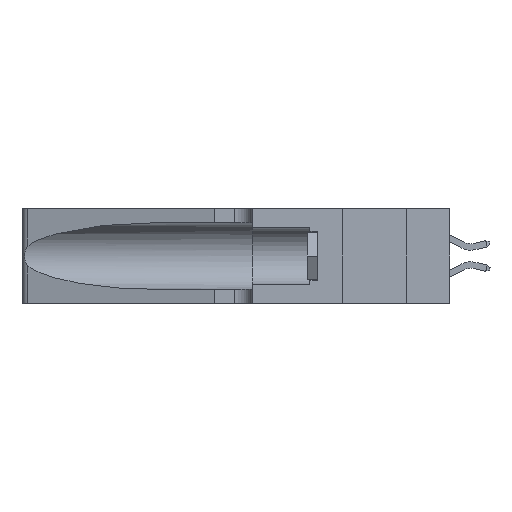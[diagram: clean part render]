
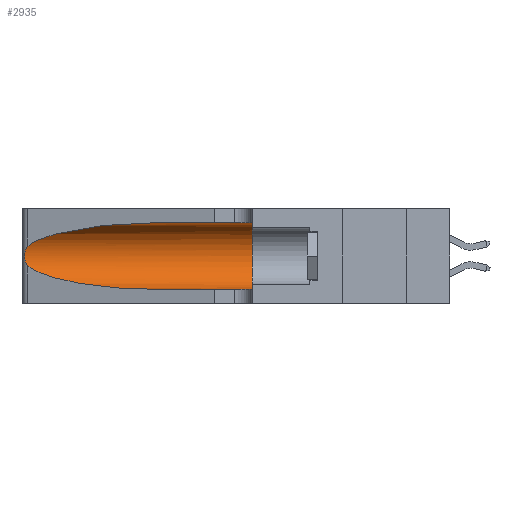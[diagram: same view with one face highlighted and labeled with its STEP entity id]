
A CAD part, left-side view. The second image highlights one B-rep face of the part: STEP entity #2935.
In plain terms, the highlighted cylindrical face has radius 3.308 mm (diameter 6.617 mm), a partial arc.
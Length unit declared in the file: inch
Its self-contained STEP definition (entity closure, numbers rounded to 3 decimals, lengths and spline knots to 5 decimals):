
#1619 = LINE ( 'NONE', #12728, #6188 ) ;
#2075 = CARTESIAN_POINT ( 'NONE',  ( 0.1305, 0.72297, 0.31525 ) ) ;
#2179 = CARTESIAN_POINT ( 'NONE',  ( 0.25789, 1.23486, 0.15765 ) ) ;
#2446 = CARTESIAN_POINT ( 'NONE',  ( 0.26075, 1.23896, 0.178 ) ) ;
#2935 = ADVANCED_FACE ( 'NONE', ( #6365 ), #4910, .F. ) ;
#4309 = CARTESIAN_POINT ( 'NONE',  ( 0.25487, 1.22718, 0.14631 ) ) ;
#4495 = B_SPLINE_CURVE_WITH_KNOTS ( 'NONE', 3,
 ( #8380, #15113, #19557, #6216, #22036, #8660, #22230, #2446, #17710, #15589, #2179, #4598, #26630, #6900 ),
 .UNSPECIFIED., .F., .F.,
 ( 4, 2, 2, 2, 2, 2, 4 ),
 ( 0., 0.00027, 0.00053, 0.00107, 0.0016, 0.00187, 0.00214 ),
 .UNSPECIFIED. ) ;
#4539 = ORIENTED_EDGE ( 'NONE', *, *, #16274, .T. ) ;
#4574 = DIRECTION ( 'NONE',  ( 0., -1., 0. ) ) ;
#4598 = CARTESIAN_POINT ( 'NONE',  ( 0.25639, 1.23186, 0.15144 ) ) ;
#4760 = DIRECTION ( 'NONE',  ( 0., 0., -1. ) ) ;
#4910 = CYLINDRICAL_SURFACE ( 'NONE', #7847, 0.13025 ) ;
#5083 = CARTESIAN_POINT ( 'NONE',  ( 0.25487, 1.22718, 0.22369 ) ) ;
#5409 = CARTESIAN_POINT ( 'NONE',  ( 0.2373, 1.15595, 0.28018 ) ) ;
#5588 = VERTEX_POINT ( 'NONE', #21264 ) ;
#6188 = VECTOR ( 'NONE', #12438, 39.37008 ) ;
#6216 = CARTESIAN_POINT ( 'NONE',  ( 0.25787, 1.23484, 0.2124 ) ) ;
#6365 = FACE_OUTER_BOUND ( 'NONE', #6972, .T. ) ;
#6838 = DIRECTION ( 'NONE',  ( 0., 0., 1. ) ) ;
#6900 = CARTESIAN_POINT ( 'NONE',  ( 0.25487, 1.22718, 0.14631 ) ) ;
#6972 = EDGE_LOOP ( 'NONE', ( #18637, #4539, #15018, #19107, #23450, #9106 ) ) ;
#7404 = DIRECTION ( 'NONE',  ( 0., -1., 0. ) ) ;
#7590 =( BOUNDED_CURVE ( )  B_SPLINE_CURVE ( 3, ( #9832, #14424, #5409, #21151 ),
 .UNSPECIFIED., .F., .T. ) 
 B_SPLINE_CURVE_WITH_KNOTS ( ( 4, 4 ),
 ( 1.5708, 2.84003 ),
 .UNSPECIFIED. ) 
 CURVE ( )  GEOMETRIC_REPRESENTATION_ITEM ( )  RATIONAL_B_SPLINE_CURVE ( ( 1., 0.87, 0.87, 1. ) ) 
 REPRESENTATION_ITEM ( '' )  );
#7847 = AXIS2_PLACEMENT_3D ( 'NONE', #18058, #4574, #4760 ) ;
#8380 = CARTESIAN_POINT ( 'NONE',  ( 0.25487, 1.22718, 0.22369 ) ) ;
#8660 = CARTESIAN_POINT ( 'NONE',  ( 0.26018, 1.23835, 0.19895 ) ) ;
#9106 = ORIENTED_EDGE ( 'NONE', *, *, #10379, .F. ) ;
#9832 = CARTESIAN_POINT ( 'NONE',  ( 0.1305, 0.72297, 0.31525 ) ) ;
#10379 = EDGE_CURVE ( 'NONE', #26397, #13782, #1619, .T. ) ;
#12438 = DIRECTION ( 'NONE',  ( 0., -1., 0. ) ) ;
#12728 = CARTESIAN_POINT ( 'NONE',  ( 0.1305, 1.61858, 0.31525 ) ) ;
#12805 = VERTEX_POINT ( 'NONE', #5083 ) ;
#12950 = EDGE_CURVE ( 'NONE', #26397, #12805, #7590, .T. ) ;
#13387 = DIRECTION ( 'NONE',  ( 0., 1., 0. ) ) ;
#13565 = CARTESIAN_POINT ( 'NONE',  ( 0.1305, 0.35, 0.185 ) ) ;
#13782 = VERTEX_POINT ( 'NONE', #26736 ) ;
#14424 = CARTESIAN_POINT ( 'NONE',  ( 0.18966, 0.96281, 0.31525 ) ) ;
#14472 = LINE ( 'NONE', #23222, #14848 ) ;
#14848 = VECTOR ( 'NONE', #7404, 39.37008 ) ;
#14995 = CARTESIAN_POINT ( 'NONE',  ( 0.1305, 0.72297, 0.05475 ) ) ;
#15018 = ORIENTED_EDGE ( 'NONE', *, *, #19377, .T. ) ;
#15113 = CARTESIAN_POINT ( 'NONE',  ( 0.25555, 1.22994, 0.2215 ) ) ;
#15589 = CARTESIAN_POINT ( 'NONE',  ( 0.25856, 1.23593, 0.16098 ) ) ;
#16274 = EDGE_CURVE ( 'NONE', #12805, #27857, #4495, .T. ) ;
#17016 = AXIS2_PLACEMENT_3D ( 'NONE', #13565, #13387, #6838 ) ;
#17710 = CARTESIAN_POINT ( 'NONE',  ( 0.26017, 1.23833, 0.17102 ) ) ;
#18058 = CARTESIAN_POINT ( 'NONE',  ( 0.1305, 1.61858, 0.185 ) ) ;
#18637 = ORIENTED_EDGE ( 'NONE', *, *, #12950, .T. ) ;
#19107 = ORIENTED_EDGE ( 'NONE', *, *, #21839, .T. ) ;
#19377 = EDGE_CURVE ( 'NONE', #27857, #5588, #28364, .T. ) ;
#19450 = CARTESIAN_POINT ( 'NONE',  ( 0.25487, 1.22718, 0.14631 ) ) ;
#19557 = CARTESIAN_POINT ( 'NONE',  ( 0.25639, 1.23184, 0.21858 ) ) ;
#21151 = CARTESIAN_POINT ( 'NONE',  ( 0.25487, 1.22718, 0.22369 ) ) ;
#21264 = CARTESIAN_POINT ( 'NONE',  ( 0.1305, 0.72297, 0.05475 ) ) ;
#21446 = CARTESIAN_POINT ( 'NONE',  ( 0.1305, 0.35, 0.05475 ) ) ;
#21839 = EDGE_CURVE ( 'NONE', #5588, #26100, #14472, .T. ) ;
#22036 = CARTESIAN_POINT ( 'NONE',  ( 0.25854, 1.2359, 0.20912 ) ) ;
#22230 = CARTESIAN_POINT ( 'NONE',  ( 0.26075, 1.23896, 0.19203 ) ) ;
#22276 = CIRCLE ( 'NONE', #17016, 0.13025 ) ;
#23222 = CARTESIAN_POINT ( 'NONE',  ( 0.1305, 1.61858, 0.05475 ) ) ;
#23450 = ORIENTED_EDGE ( 'NONE', *, *, #23656, .F. ) ;
#23656 = EDGE_CURVE ( 'NONE', #13782, #26100, #22276, .T. ) ;
#26100 = VERTEX_POINT ( 'NONE', #21446 ) ;
#26212 = CARTESIAN_POINT ( 'NONE',  ( 0.18966, 0.96281, 0.05475 ) ) ;
#26319 = CARTESIAN_POINT ( 'NONE',  ( 0.2373, 1.15595, 0.08982 ) ) ;
#26397 = VERTEX_POINT ( 'NONE', #2075 ) ;
#26630 = CARTESIAN_POINT ( 'NONE',  ( 0.25555, 1.22993, 0.14849 ) ) ;
#26736 = CARTESIAN_POINT ( 'NONE',  ( 0.1305, 0.35, 0.31525 ) ) ;
#27857 = VERTEX_POINT ( 'NONE', #4309 ) ;
#28364 =( BOUNDED_CURVE ( )  B_SPLINE_CURVE ( 3, ( #19450, #26319, #26212, #14995 ),
 .UNSPECIFIED., .F., .T. ) 
 B_SPLINE_CURVE_WITH_KNOTS ( ( 4, 4 ),
 ( 3.44316, 4.71239 ),
 .UNSPECIFIED. ) 
 CURVE ( )  GEOMETRIC_REPRESENTATION_ITEM ( )  RATIONAL_B_SPLINE_CURVE ( ( 1., 0.87, 0.87, 1. ) ) 
 REPRESENTATION_ITEM ( '' )  );
